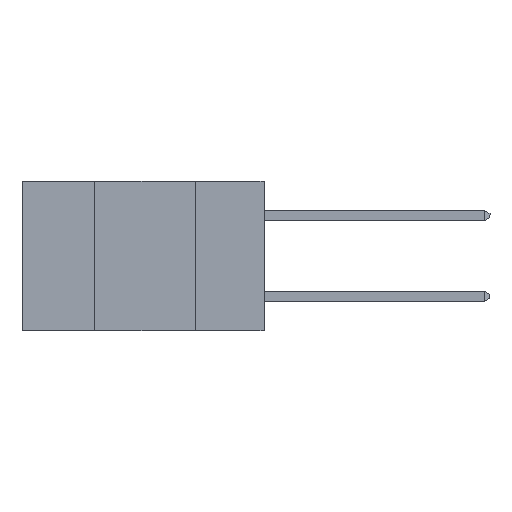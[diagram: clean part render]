
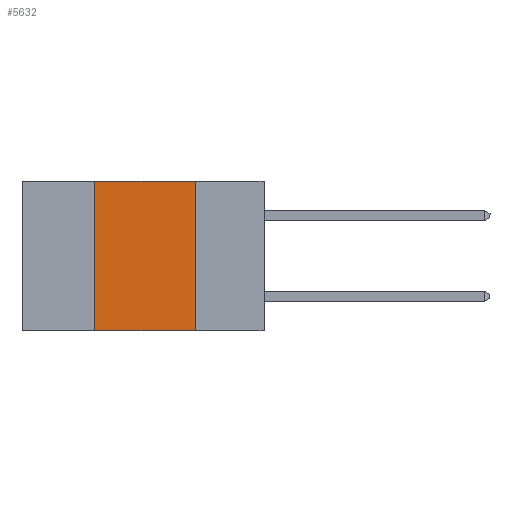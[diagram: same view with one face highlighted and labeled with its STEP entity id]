
A CAD part, left-side view. The second image highlights one B-rep face of the part: STEP entity #5632.
In plain terms, the highlighted planar face has unit normal (-1, 0, 0).
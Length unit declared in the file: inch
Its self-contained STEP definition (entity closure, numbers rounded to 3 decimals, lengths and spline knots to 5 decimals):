
#358 = VERTEX_POINT ( 'NONE', #11469 ) ;
#894 = ORIENTED_EDGE ( 'NONE', *, *, #6137, .F. ) ;
#1003 = DIRECTION ( 'NONE',  ( 0., 0., 1. ) ) ;
#1148 = ORIENTED_EDGE ( 'NONE', *, *, #17345, .T. ) ;
#1211 = LINE ( 'NONE', #16737, #9125 ) ;
#1344 = PLANE ( 'NONE',  #10463 ) ;
#1825 = DIRECTION ( 'NONE',  ( 0., -1., 0. ) ) ;
#2637 = ORIENTED_EDGE ( 'NONE', *, *, #14409, .F. ) ;
#2795 = DIRECTION ( 'NONE',  ( 1., 0., 0. ) ) ;
#3556 = EDGE_LOOP ( 'NONE', ( #2637, #6440, #894, #1148 ) ) ;
#4588 = EDGE_CURVE ( 'NONE', #358, #14882, #9624, .T. ) ;
#5284 = CARTESIAN_POINT ( 'NONE',  ( 0., 0.42, 0. ) ) ;
#5632 = ADVANCED_FACE ( 'NONE', ( #10649 ), #1344, .F. ) ;
#6137 = EDGE_CURVE ( 'NONE', #13025, #358, #16844, .T. ) ;
#6440 = ORIENTED_EDGE ( 'NONE', *, *, #4588, .F. ) ;
#6503 = VECTOR ( 'NONE', #1003, 39.37008 ) ;
#7449 = CARTESIAN_POINT ( 'NONE',  ( 0., 0.17, 0. ) ) ;
#7498 = VERTEX_POINT ( 'NONE', #11000 ) ;
#7798 = DIRECTION ( 'NONE',  ( 0., 0., -1. ) ) ;
#9125 = VECTOR ( 'NONE', #15463, 39.37008 ) ;
#9624 = LINE ( 'NONE', #16400, #13640 ) ;
#10463 = AXIS2_PLACEMENT_3D ( 'NONE', #11116, #2795, #12465 ) ;
#10649 = FACE_OUTER_BOUND ( 'NONE', #3556, .T. ) ;
#11000 = CARTESIAN_POINT ( 'NONE',  ( 0., 0.17, -0.37 ) ) ;
#11116 = CARTESIAN_POINT ( 'NONE',  ( 0., 0.6, 0. ) ) ;
#11469 = CARTESIAN_POINT ( 'NONE',  ( 0., 0.42, 0. ) ) ;
#12465 = DIRECTION ( 'NONE',  ( 0., 0., -1. ) ) ;
#13025 = VERTEX_POINT ( 'NONE', #16294 ) ;
#13640 = VECTOR ( 'NONE', #1825, 39.37008 ) ;
#13897 = LINE ( 'NONE', #15882, #14444 ) ;
#14409 = EDGE_CURVE ( 'NONE', #14882, #7498, #13897, .T. ) ;
#14444 = VECTOR ( 'NONE', #7798, 39.37008 ) ;
#14882 = VERTEX_POINT ( 'NONE', #7449 ) ;
#15463 = DIRECTION ( 'NONE',  ( 0., -1., 0. ) ) ;
#15882 = CARTESIAN_POINT ( 'NONE',  ( 0., 0.17, 0. ) ) ;
#16294 = CARTESIAN_POINT ( 'NONE',  ( 0., 0.42, -0.37 ) ) ;
#16400 = CARTESIAN_POINT ( 'NONE',  ( 0., 0.6, 0. ) ) ;
#16737 = CARTESIAN_POINT ( 'NONE',  ( 0., 0.6, -0.37 ) ) ;
#16844 = LINE ( 'NONE', #5284, #6503 ) ;
#17345 = EDGE_CURVE ( 'NONE', #13025, #7498, #1211, .T. ) ;
